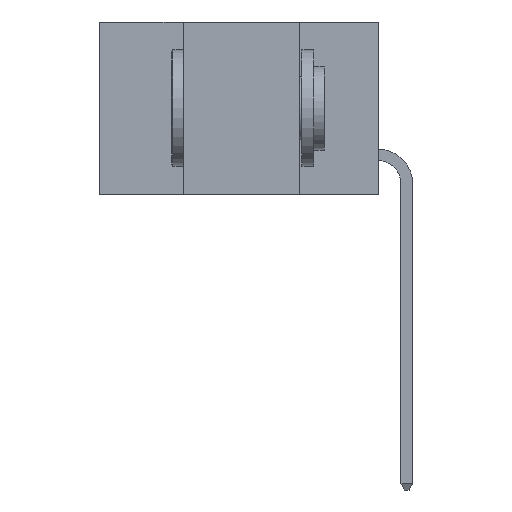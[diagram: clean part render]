
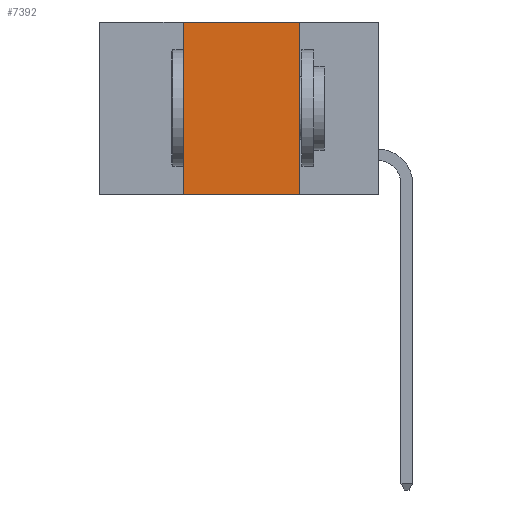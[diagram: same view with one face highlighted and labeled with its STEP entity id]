
A CAD part, left-side view. The second image highlights one B-rep face of the part: STEP entity #7392.
In plain terms, the highlighted planar face has unit normal (-1, 0, 0).
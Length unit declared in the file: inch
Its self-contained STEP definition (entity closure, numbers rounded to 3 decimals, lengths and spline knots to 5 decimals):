
#688 = LINE ( 'NONE', #15954, #20493 ) ;
#903 = ORIENTED_EDGE ( 'NONE', *, *, #1052, .F. ) ;
#1052 = EDGE_CURVE ( 'NONE', #7478, #9563, #688, .T. ) ;
#1323 = DIRECTION ( 'NONE',  ( 0., -1., 0. ) ) ;
#2114 = VECTOR ( 'NONE', #1323, 39.37008 ) ;
#3560 = VERTEX_POINT ( 'NONE', #15449 ) ;
#4117 = ORIENTED_EDGE ( 'NONE', *, *, #19860, .F. ) ;
#4190 = EDGE_CURVE ( 'NONE', #3560, #12035, #4600, .T. ) ;
#4255 = CARTESIAN_POINT ( 'NONE',  ( 0., 0.17, -0.37 ) ) ;
#4600 = LINE ( 'NONE', #17733, #16880 ) ;
#5093 = LINE ( 'NONE', #11843, #13099 ) ;
#7392 = ADVANCED_FACE ( 'NONE', ( #11733 ), #18307, .F. ) ;
#7478 = VERTEX_POINT ( 'NONE', #16421 ) ;
#8723 = DIRECTION ( 'NONE',  ( 0., -1., 0. ) ) ;
#9163 = AXIS2_PLACEMENT_3D ( 'NONE', #18873, #18149, #18123 ) ;
#9563 = VERTEX_POINT ( 'NONE', #12322 ) ;
#10902 = ORIENTED_EDGE ( 'NONE', *, *, #4190, .F. ) ;
#11733 = FACE_OUTER_BOUND ( 'NONE', #17264, .T. ) ;
#11843 = CARTESIAN_POINT ( 'NONE',  ( 0., 0.6, 0. ) ) ;
#12035 = VERTEX_POINT ( 'NONE', #4255 ) ;
#12071 = ORIENTED_EDGE ( 'NONE', *, *, #19149, .T. ) ;
#12322 = CARTESIAN_POINT ( 'NONE',  ( 0., 0.42, 0. ) ) ;
#12551 = CARTESIAN_POINT ( 'NONE',  ( 0., 0.6, -0.37 ) ) ;
#13099 = VECTOR ( 'NONE', #8723, 39.37008 ) ;
#15449 = CARTESIAN_POINT ( 'NONE',  ( 0., 0.17, 0. ) ) ;
#15954 = CARTESIAN_POINT ( 'NONE',  ( 0., 0.42, -0.37 ) ) ;
#16260 = DIRECTION ( 'NONE',  ( 0., 0., 1. ) ) ;
#16421 = CARTESIAN_POINT ( 'NONE',  ( 0., 0.42, -0.37 ) ) ;
#16880 = VECTOR ( 'NONE', #17657, 39.37008 ) ;
#17264 = EDGE_LOOP ( 'NONE', ( #10902, #4117, #903, #12071 ) ) ;
#17657 = DIRECTION ( 'NONE',  ( 0., 0., -1. ) ) ;
#17733 = CARTESIAN_POINT ( 'NONE',  ( 0., 0.17, -0.37 ) ) ;
#18123 = DIRECTION ( 'NONE',  ( 0., 0., -1. ) ) ;
#18149 = DIRECTION ( 'NONE',  ( 1., 0., 0. ) ) ;
#18161 = LINE ( 'NONE', #12551, #2114 ) ;
#18307 = PLANE ( 'NONE',  #9163 ) ;
#18873 = CARTESIAN_POINT ( 'NONE',  ( 0., 0.6, 0. ) ) ;
#19149 = EDGE_CURVE ( 'NONE', #7478, #12035, #18161, .T. ) ;
#19860 = EDGE_CURVE ( 'NONE', #9563, #3560, #5093, .T. ) ;
#20493 = VECTOR ( 'NONE', #16260, 39.37008 ) ;
